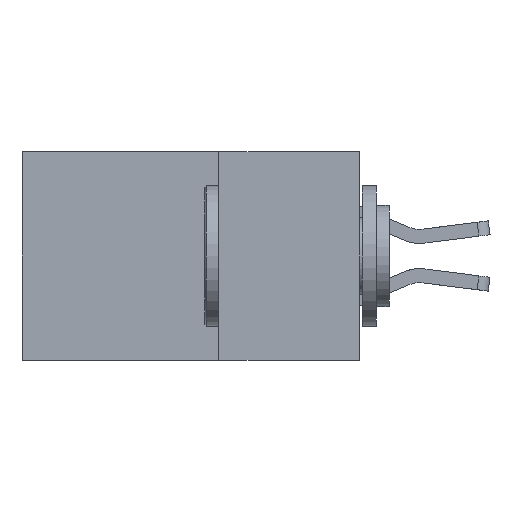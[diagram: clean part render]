
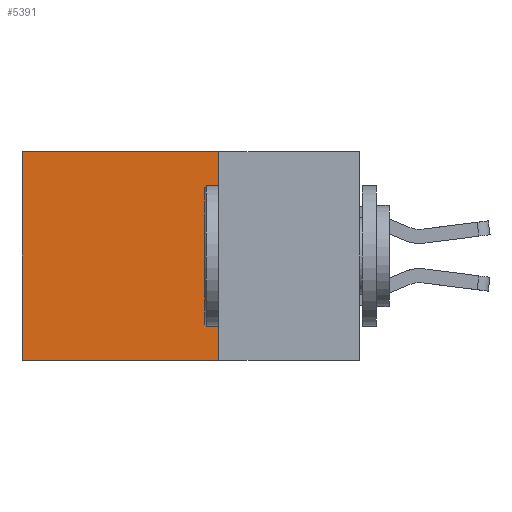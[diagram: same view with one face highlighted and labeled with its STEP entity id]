
A CAD part, left-side view. The second image highlights one B-rep face of the part: STEP entity #5391.
In plain terms, the highlighted planar face has unit normal (-1, 0, 0).
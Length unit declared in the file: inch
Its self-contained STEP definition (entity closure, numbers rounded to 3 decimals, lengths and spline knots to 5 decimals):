
#153 = DIRECTION ( 'NONE',  ( 0., 0., -1. ) ) ;
#177 = DIRECTION ( 'NONE',  ( 0., 1., 0. ) ) ;
#742 = EDGE_CURVE ( 'NONE', #2258, #7705, #8264, .T. ) ;
#844 = CARTESIAN_POINT ( 'NONE',  ( 0.2875, 0.25, 0. ) ) ;
#1088 = LINE ( 'NONE', #10768, #9745 ) ;
#1148 = LINE ( 'NONE', #4420, #7822 ) ;
#1819 = CARTESIAN_POINT ( 'NONE',  ( 0.2875, 0.25, -0.37 ) ) ;
#2258 = VERTEX_POINT ( 'NONE', #844 ) ;
#2594 = CARTESIAN_POINT ( 'NONE',  ( 0.2875, 0.25, 0. ) ) ;
#2995 = VECTOR ( 'NONE', #9484, 39.37008 ) ;
#3825 = CARTESIAN_POINT ( 'NONE',  ( 0.2875, 0.25, 0. ) ) ;
#3992 = FACE_OUTER_BOUND ( 'NONE', #6831, .T. ) ;
#4420 = CARTESIAN_POINT ( 'NONE',  ( 0.2875, 0.6, 0. ) ) ;
#4656 = EDGE_CURVE ( 'NONE', #7705, #9912, #1088, .T. ) ;
#5098 = CARTESIAN_POINT ( 'NONE',  ( 0.2875, 0.6, 0. ) ) ;
#5391 = ADVANCED_FACE ( 'NONE', ( #3992 ), #7375, .F. ) ;
#5601 = ORIENTED_EDGE ( 'NONE', *, *, #742, .F. ) ;
#5937 = VERTEX_POINT ( 'NONE', #5098 ) ;
#6084 = VECTOR ( 'NONE', #153, 39.37008 ) ;
#6831 = EDGE_LOOP ( 'NONE', ( #7038, #7286, #5601, #8081 ) ) ;
#7038 = ORIENTED_EDGE ( 'NONE', *, *, #7655, .T. ) ;
#7142 = CARTESIAN_POINT ( 'NONE',  ( 0.2875, 0.6, -0.37 ) ) ;
#7286 = ORIENTED_EDGE ( 'NONE', *, *, #4656, .F. ) ;
#7375 = PLANE ( 'NONE',  #9650 ) ;
#7460 = DIRECTION ( 'NONE',  ( 0., 0., -1. ) ) ;
#7481 = DIRECTION ( 'NONE',  ( 1., 0., 0. ) ) ;
#7493 = CARTESIAN_POINT ( 'NONE',  ( 0.2875, 0.25, 0. ) ) ;
#7655 = EDGE_CURVE ( 'NONE', #5937, #9912, #1148, .T. ) ;
#7705 = VERTEX_POINT ( 'NONE', #1819 ) ;
#7822 = VECTOR ( 'NONE', #7851, 39.37008 ) ;
#7851 = DIRECTION ( 'NONE',  ( 0., 0., -1. ) ) ;
#8081 = ORIENTED_EDGE ( 'NONE', *, *, #9768, .T. ) ;
#8264 = LINE ( 'NONE', #3825, #6084 ) ;
#9484 = DIRECTION ( 'NONE',  ( 0., 1., 0. ) ) ;
#9650 = AXIS2_PLACEMENT_3D ( 'NONE', #7493, #7481, #7460 ) ;
#9745 = VECTOR ( 'NONE', #177, 39.37008 ) ;
#9768 = EDGE_CURVE ( 'NONE', #2258, #5937, #9836, .T. ) ;
#9836 = LINE ( 'NONE', #2594, #2995 ) ;
#9912 = VERTEX_POINT ( 'NONE', #7142 ) ;
#10768 = CARTESIAN_POINT ( 'NONE',  ( 0.2875, 0.25, -0.37 ) ) ;
